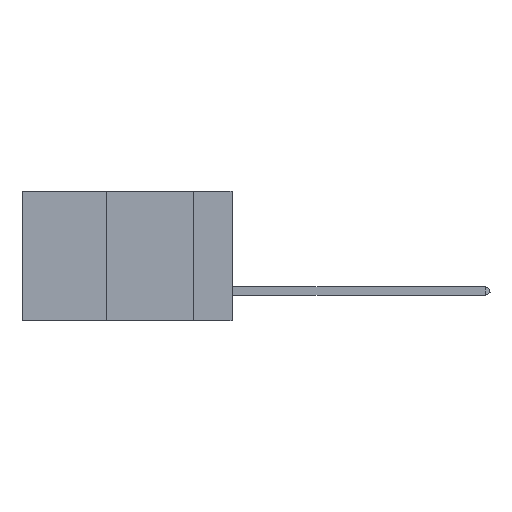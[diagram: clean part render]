
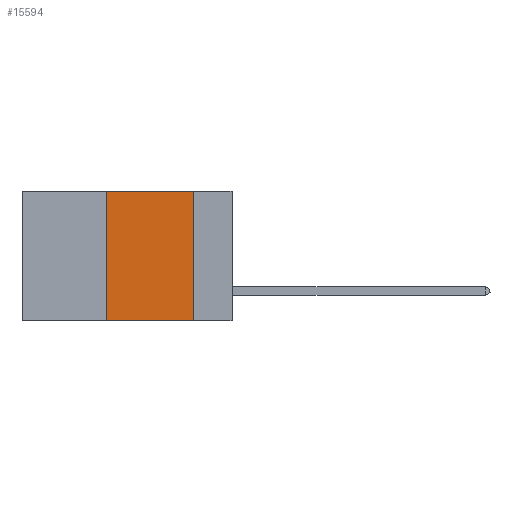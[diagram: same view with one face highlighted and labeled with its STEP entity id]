
A CAD part, left-side view. The second image highlights one B-rep face of the part: STEP entity #15594.
In plain terms, the highlighted planar face has unit normal (-1, 0, 0).
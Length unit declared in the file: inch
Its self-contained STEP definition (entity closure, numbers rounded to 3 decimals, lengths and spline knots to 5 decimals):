
#696 = DIRECTION ( 'NONE',  ( 0., 0., -1. ) ) ;
#1015 = EDGE_CURVE ( 'NONE', #4183, #16488, #15473, .T. ) ;
#1116 = VECTOR ( 'NONE', #15611, 39.37008 ) ;
#1395 = EDGE_CURVE ( 'NONE', #4183, #19543, #17061, .T. ) ;
#1723 = VECTOR ( 'NONE', #696, 39.37008 ) ;
#2306 = VECTOR ( 'NONE', #4654, 39.37008 ) ;
#3042 = DIRECTION ( 'NONE',  ( 1., 0., 0. ) ) ;
#4183 = VERTEX_POINT ( 'NONE', #18451 ) ;
#4654 = DIRECTION ( 'NONE',  ( 0., -1., 0. ) ) ;
#4720 = CARTESIAN_POINT ( 'NONE',  ( 0., 0.6, 0. ) ) ;
#4781 = DIRECTION ( 'NONE',  ( 0., 0., -1. ) ) ;
#5973 = CARTESIAN_POINT ( 'NONE',  ( 0., 0.11, 0. ) ) ;
#7832 = ORIENTED_EDGE ( 'NONE', *, *, #1015, .T. ) ;
#8849 = LINE ( 'NONE', #12150, #1723 ) ;
#9914 = EDGE_CURVE ( 'NONE', #13987, #16488, #8849, .T. ) ;
#10110 = CARTESIAN_POINT ( 'NONE',  ( 0., 0.36, 0. ) ) ;
#11364 = LINE ( 'NONE', #15534, #1116 ) ;
#11796 = DIRECTION ( 'NONE',  ( 0., 0., 1. ) ) ;
#12126 = EDGE_CURVE ( 'NONE', #19543, #13987, #11364, .T. ) ;
#12150 = CARTESIAN_POINT ( 'NONE',  ( 0., 0.11, 0. ) ) ;
#12199 = CARTESIAN_POINT ( 'NONE',  ( 0., 0.11, -0.37 ) ) ;
#12223 = ORIENTED_EDGE ( 'NONE', *, *, #9914, .F. ) ;
#12680 = FACE_OUTER_BOUND ( 'NONE', #16591, .T. ) ;
#13051 = CARTESIAN_POINT ( 'NONE',  ( 0., 0.6, -0.37 ) ) ;
#13200 = PLANE ( 'NONE',  #16627 ) ;
#13987 = VERTEX_POINT ( 'NONE', #5973 ) ;
#15473 = LINE ( 'NONE', #13051, #2306 ) ;
#15534 = CARTESIAN_POINT ( 'NONE',  ( 0., 0.6, 0. ) ) ;
#15594 = ADVANCED_FACE ( 'NONE', ( #12680 ), #13200, .F. ) ;
#15611 = DIRECTION ( 'NONE',  ( 0., -1., 0. ) ) ;
#16488 = VERTEX_POINT ( 'NONE', #12199 ) ;
#16591 = EDGE_LOOP ( 'NONE', ( #12223, #20312, #20063, #7832 ) ) ;
#16627 = AXIS2_PLACEMENT_3D ( 'NONE', #4720, #3042, #4781 ) ;
#17061 = LINE ( 'NONE', #10110, #20470 ) ;
#18451 = CARTESIAN_POINT ( 'NONE',  ( 0., 0.36, -0.37 ) ) ;
#19427 = CARTESIAN_POINT ( 'NONE',  ( 0., 0.36, 0. ) ) ;
#19543 = VERTEX_POINT ( 'NONE', #19427 ) ;
#20063 = ORIENTED_EDGE ( 'NONE', *, *, #1395, .F. ) ;
#20312 = ORIENTED_EDGE ( 'NONE', *, *, #12126, .F. ) ;
#20470 = VECTOR ( 'NONE', #11796, 39.37008 ) ;
